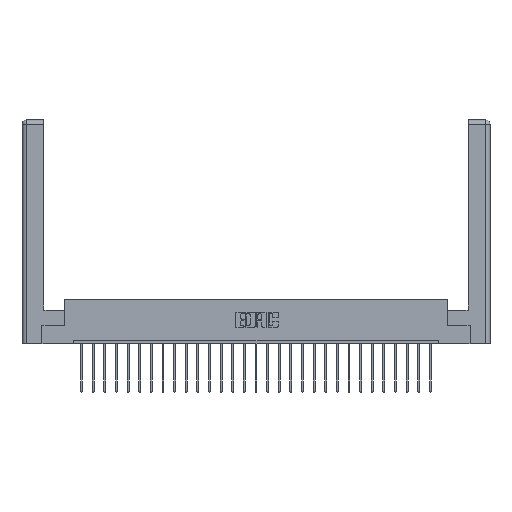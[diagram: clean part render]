
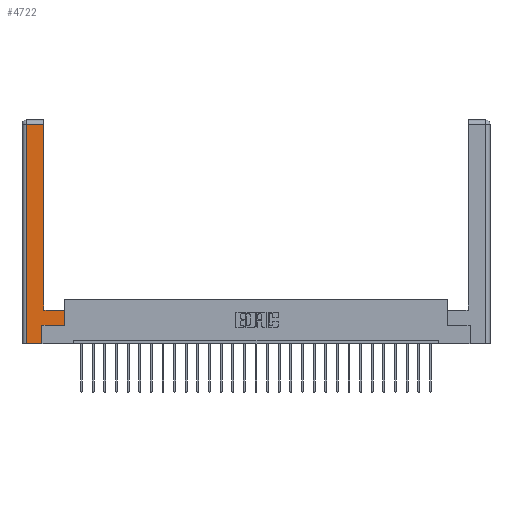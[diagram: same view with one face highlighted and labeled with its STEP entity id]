
A CAD part, top view. The second image highlights one B-rep face of the part: STEP entity #4722.
In plain terms, the highlighted planar face has unit normal (0, 0, 1).
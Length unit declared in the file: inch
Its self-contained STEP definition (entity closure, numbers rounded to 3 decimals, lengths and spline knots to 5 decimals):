
#39 = EDGE_CURVE ( 'NONE', #2880, #26686, #26035, .T. ) ;
#558 = CARTESIAN_POINT ( 'NONE',  ( 0.295, 3., 0. ) ) ;
#586 = VECTOR ( 'NONE', #2558, 39.37008 ) ;
#1671 = VECTOR ( 'NONE', #10076, 39.37008 ) ;
#1971 = VERTEX_POINT ( 'NONE', #14283 ) ;
#2120 = VECTOR ( 'NONE', #11901, 39.37008 ) ;
#2337 = DIRECTION ( 'NONE',  ( -1., 0., 0. ) ) ;
#2558 = DIRECTION ( 'NONE',  ( -1., 0., 0. ) ) ;
#2880 = VERTEX_POINT ( 'NONE', #23238 ) ;
#4413 = CARTESIAN_POINT ( 'NONE',  ( 0.0615, 2.94, 0. ) ) ;
#4535 = CARTESIAN_POINT ( 'NONE',  ( 0.295, 0.45, 0. ) ) ;
#4721 = EDGE_CURVE ( 'NONE', #7945, #1971, #17716, .T. ) ;
#4722 = ADVANCED_FACE ( 'NONE', ( #10506 ), #9707, .F. ) ;
#4821 = LINE ( 'NONE', #4413, #586 ) ;
#5289 = ORIENTED_EDGE ( 'NONE', *, *, #21244, .T. ) ;
#5449 = VERTEX_POINT ( 'NONE', #20908 ) ;
#5985 = CARTESIAN_POINT ( 'NONE',  ( 0.295, 2.94, 0. ) ) ;
#6985 = ORIENTED_EDGE ( 'NONE', *, *, #26836, .T. ) ;
#7092 = VECTOR ( 'NONE', #21968, 39.37008 ) ;
#7300 = ORIENTED_EDGE ( 'NONE', *, *, #4721, .T. ) ;
#7599 = DIRECTION ( 'NONE',  ( 0., 0., -1. ) ) ;
#7688 = CARTESIAN_POINT ( 'NONE',  ( 0.265, 0.245, 0. ) ) ;
#7945 = VERTEX_POINT ( 'NONE', #16058 ) ;
#9039 = LINE ( 'NONE', #25805, #7092 ) ;
#9304 = DIRECTION ( 'NONE',  ( 0., 1., 0. ) ) ;
#9359 = VECTOR ( 'NONE', #26233, 39.37008 ) ;
#9707 = PLANE ( 'NONE',  #20084 ) ;
#9724 = CARTESIAN_POINT ( 'NONE',  ( 0.0615, 0., 0. ) ) ;
#9859 = VECTOR ( 'NONE', #16221, 39.37008 ) ;
#10076 = DIRECTION ( 'NONE',  ( 1., 0., 0. ) ) ;
#10506 = FACE_OUTER_BOUND ( 'NONE', #20135, .T. ) ;
#11095 = VECTOR ( 'NONE', #2337, 39.37008 ) ;
#11901 = DIRECTION ( 'NONE',  ( 0., 1., 0. ) ) ;
#11997 = LINE ( 'NONE', #9724, #9359 ) ;
#12573 = VECTOR ( 'NONE', #9304, 39.37008 ) ;
#13220 = LINE ( 'NONE', #7688, #2120 ) ;
#13341 = ORIENTED_EDGE ( 'NONE', *, *, #13563, .T. ) ;
#13384 = LINE ( 'NONE', #4535, #11095 ) ;
#13446 = ORIENTED_EDGE ( 'NONE', *, *, #39, .T. ) ;
#13563 = EDGE_CURVE ( 'NONE', #5449, #2880, #13384, .T. ) ;
#13844 = ORIENTED_EDGE ( 'NONE', *, *, #16864, .T. ) ;
#13999 = CARTESIAN_POINT ( 'NONE',  ( 0., 0., 0. ) ) ;
#14283 = CARTESIAN_POINT ( 'NONE',  ( 0.265, 0., 0. ) ) ;
#15581 = CARTESIAN_POINT ( 'NONE',  ( 0.265, 0., 0. ) ) ;
#15694 = VERTEX_POINT ( 'NONE', #15723 ) ;
#15709 = ORIENTED_EDGE ( 'NONE', *, *, #18442, .T. ) ;
#15716 = EDGE_CURVE ( 'NONE', #17876, #5449, #9039, .T. ) ;
#15723 = CARTESIAN_POINT ( 'NONE',  ( 0.265, 0.245, 0. ) ) ;
#16058 = CARTESIAN_POINT ( 'NONE',  ( 0.0615, 0., 0. ) ) ;
#16221 = DIRECTION ( 'NONE',  ( 1., 0., 0. ) ) ;
#16864 = EDGE_CURVE ( 'NONE', #1971, #15694, #13220, .T. ) ;
#17716 = LINE ( 'NONE', #15581, #9859 ) ;
#17876 = VERTEX_POINT ( 'NONE', #21873 ) ;
#17980 = CARTESIAN_POINT ( 'NONE',  ( 0.0615, 2.94, 0. ) ) ;
#18040 = LINE ( 'NONE', #26810, #1671 ) ;
#18442 = EDGE_CURVE ( 'NONE', #15694, #17876, #18040, .T. ) ;
#18993 = ORIENTED_EDGE ( 'NONE', *, *, #15716, .T. ) ;
#20084 = AXIS2_PLACEMENT_3D ( 'NONE', #13999, #7599, #20240 ) ;
#20135 = EDGE_LOOP ( 'NONE', ( #13446, #6985, #5289, #7300, #13844, #15709, #18993, #13341 ) ) ;
#20240 = DIRECTION ( 'NONE',  ( -1., 0., 0. ) ) ;
#20908 = CARTESIAN_POINT ( 'NONE',  ( 0.565, 0.45, 0. ) ) ;
#21244 = EDGE_CURVE ( 'NONE', #26291, #7945, #11997, .T. ) ;
#21873 = CARTESIAN_POINT ( 'NONE',  ( 0.565, 0.245, 0. ) ) ;
#21968 = DIRECTION ( 'NONE',  ( 0., 1., 0. ) ) ;
#23238 = CARTESIAN_POINT ( 'NONE',  ( 0.295, 0.45, 0. ) ) ;
#25805 = CARTESIAN_POINT ( 'NONE',  ( 0.565, 0.45, 0. ) ) ;
#26035 = LINE ( 'NONE', #558, #12573 ) ;
#26233 = DIRECTION ( 'NONE',  ( 0., -1., 0. ) ) ;
#26291 = VERTEX_POINT ( 'NONE', #17980 ) ;
#26686 = VERTEX_POINT ( 'NONE', #5985 ) ;
#26810 = CARTESIAN_POINT ( 'NONE',  ( 0.565, 0.245, 0. ) ) ;
#26836 = EDGE_CURVE ( 'NONE', #26686, #26291, #4821, .T. ) ;
